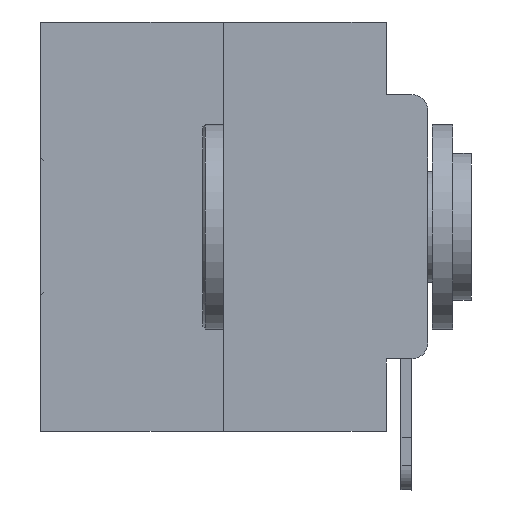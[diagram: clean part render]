
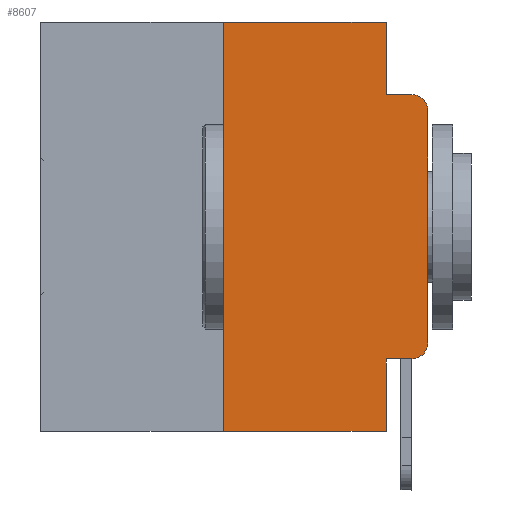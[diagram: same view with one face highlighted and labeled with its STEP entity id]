
A CAD part, left-side view. The second image highlights one B-rep face of the part: STEP entity #8607.
In plain terms, the highlighted planar face has unit normal (-1, 0, 0).
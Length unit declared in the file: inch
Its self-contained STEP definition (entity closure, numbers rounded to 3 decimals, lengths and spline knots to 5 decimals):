
#262 = DIRECTION ( 'NONE',  ( 0., 0., -1. ) ) ;
#319 = CARTESIAN_POINT ( 'NONE',  ( 0., 0.051, -0.4115 ) ) ;
#402 = FACE_OUTER_BOUND ( 'NONE', #17905, .T. ) ;
#576 = LINE ( 'NONE', #646, #9489 ) ;
#646 = CARTESIAN_POINT ( 'NONE',  ( 0., 0.051, -0.0885 ) ) ;
#728 = DIRECTION ( 'NONE',  ( 0., 0., -1. ) ) ;
#1048 = ORIENTED_EDGE ( 'NONE', *, *, #15863, .F. ) ;
#1178 = EDGE_CURVE ( 'NONE', #18117, #3044, #16534, .T. ) ;
#1438 = CARTESIAN_POINT ( 'NONE',  ( 0., 0.25, 0. ) ) ;
#1987 = CARTESIAN_POINT ( 'NONE',  ( 0., 0., -0.1085 ) ) ;
#3044 = VERTEX_POINT ( 'NONE', #31222 ) ;
#3972 = DIRECTION ( 'NONE',  ( 0., -1., 0. ) ) ;
#4255 = EDGE_CURVE ( 'NONE', #9255, #8906, #14794, .T. ) ;
#4724 = CARTESIAN_POINT ( 'NONE',  ( 0., 0.25, -0.5 ) ) ;
#5459 = ORIENTED_EDGE ( 'NONE', *, *, #26812, .T. ) ;
#5686 = DIRECTION ( 'NONE',  ( -1., 0., 0. ) ) ;
#6007 = CARTESIAN_POINT ( 'NONE',  ( 0., 0.02, -0.1085 ) ) ;
#6396 = DIRECTION ( 'NONE',  ( 0., -1., 0. ) ) ;
#6477 = CARTESIAN_POINT ( 'NONE',  ( 0., 0., -0.3915 ) ) ;
#6578 = VECTOR ( 'NONE', #6396, 39.37008 ) ;
#6749 = LINE ( 'NONE', #26304, #31237 ) ;
#7084 = DIRECTION ( 'NONE',  ( 0., 0., -1. ) ) ;
#7358 = AXIS2_PLACEMENT_3D ( 'NONE', #6007, #5686, #728 ) ;
#7733 = ORIENTED_EDGE ( 'NONE', *, *, #22072, .F. ) ;
#7742 = VECTOR ( 'NONE', #15112, 39.37008 ) ;
#8607 = ADVANCED_FACE ( 'NONE', ( #402 ), #12983, .F. ) ;
#8906 = VERTEX_POINT ( 'NONE', #23309 ) ;
#9255 = VERTEX_POINT ( 'NONE', #29209 ) ;
#9489 = VECTOR ( 'NONE', #23239, 39.37008 ) ;
#9783 = VERTEX_POINT ( 'NONE', #6477 ) ;
#9845 = CARTESIAN_POINT ( 'NONE',  ( 0., 0.02, -0.0885 ) ) ;
#10100 = VERTEX_POINT ( 'NONE', #9845 ) ;
#10131 = CARTESIAN_POINT ( 'NONE',  ( 0., 0.473, 0. ) ) ;
#10778 = ORIENTED_EDGE ( 'NONE', *, *, #4255, .F. ) ;
#11889 = AXIS2_PLACEMENT_3D ( 'NONE', #16993, #19528, #7084 ) ;
#12983 = PLANE ( 'NONE',  #27337 ) ;
#13400 = CARTESIAN_POINT ( 'NONE',  ( 0., 0.473, 0. ) ) ;
#13422 = VERTEX_POINT ( 'NONE', #15298 ) ;
#13876 = LINE ( 'NONE', #30488, #19703 ) ;
#14374 = LINE ( 'NONE', #20135, #7742 ) ;
#14794 = LINE ( 'NONE', #17835, #16333 ) ;
#15103 = ORIENTED_EDGE ( 'NONE', *, *, #26096, .T. ) ;
#15112 = DIRECTION ( 'NONE',  ( 0., 0., -1. ) ) ;
#15298 = CARTESIAN_POINT ( 'NONE',  ( 0., 0.051, 0. ) ) ;
#15502 = DIRECTION ( 'NONE',  ( 0., -1., 0. ) ) ;
#15570 = LINE ( 'NONE', #13400, #6578 ) ;
#15663 = DIRECTION ( 'NONE',  ( 0., 0., 1. ) ) ;
#15863 = EDGE_CURVE ( 'NONE', #27999, #10100, #576, .T. ) ;
#16333 = VECTOR ( 'NONE', #262, 39.37008 ) ;
#16534 = LINE ( 'NONE', #1438, #26199 ) ;
#16773 = EDGE_CURVE ( 'NONE', #9783, #29771, #13876, .T. ) ;
#16993 = CARTESIAN_POINT ( 'NONE',  ( 0., 0.02, -0.3915 ) ) ;
#17084 = EDGE_CURVE ( 'NONE', #13422, #27999, #14374, .T. ) ;
#17223 = ORIENTED_EDGE ( 'NONE', *, *, #1178, .F. ) ;
#17383 = LINE ( 'NONE', #319, #27822 ) ;
#17763 = CIRCLE ( 'NONE', #11889, 0.02 ) ;
#17835 = CARTESIAN_POINT ( 'NONE',  ( 0., 0.051, 0. ) ) ;
#17905 = EDGE_LOOP ( 'NONE', ( #20429, #27371, #1048, #22191, #7733, #17223, #5459, #10778, #30061, #15103 ) ) ;
#18117 = VERTEX_POINT ( 'NONE', #4724 ) ;
#19135 = EDGE_CURVE ( 'NONE', #29771, #10100, #30495, .T. ) ;
#19528 = DIRECTION ( 'NONE',  ( -1., 0., 0. ) ) ;
#19703 = VECTOR ( 'NONE', #15663, 39.37008 ) ;
#20135 = CARTESIAN_POINT ( 'NONE',  ( 0., 0.051, 0. ) ) ;
#20429 = ORIENTED_EDGE ( 'NONE', *, *, #16773, .T. ) ;
#22072 = EDGE_CURVE ( 'NONE', #3044, #13422, #15570, .T. ) ;
#22191 = ORIENTED_EDGE ( 'NONE', *, *, #17084, .F. ) ;
#23239 = DIRECTION ( 'NONE',  ( 0., -1., 0. ) ) ;
#23309 = CARTESIAN_POINT ( 'NONE',  ( 0., 0.051, -0.5 ) ) ;
#23918 = CARTESIAN_POINT ( 'NONE',  ( 0., 0.051, -0.0885 ) ) ;
#25320 = DIRECTION ( 'NONE',  ( 0., 0., -1. ) ) ;
#25751 = EDGE_CURVE ( 'NONE', #9255, #31777, #17383, .T. ) ;
#26096 = EDGE_CURVE ( 'NONE', #31777, #9783, #17763, .T. ) ;
#26199 = VECTOR ( 'NONE', #31258, 39.37008 ) ;
#26304 = CARTESIAN_POINT ( 'NONE',  ( 0., 0.473, -0.5 ) ) ;
#26812 = EDGE_CURVE ( 'NONE', #18117, #8906, #6749, .T. ) ;
#27337 = AXIS2_PLACEMENT_3D ( 'NONE', #10131, #29887, #25320 ) ;
#27371 = ORIENTED_EDGE ( 'NONE', *, *, #19135, .T. ) ;
#27664 = CARTESIAN_POINT ( 'NONE',  ( 0., 0.02, -0.4115 ) ) ;
#27822 = VECTOR ( 'NONE', #15502, 39.37008 ) ;
#27999 = VERTEX_POINT ( 'NONE', #23918 ) ;
#29209 = CARTESIAN_POINT ( 'NONE',  ( 0., 0.051, -0.4115 ) ) ;
#29771 = VERTEX_POINT ( 'NONE', #1987 ) ;
#29887 = DIRECTION ( 'NONE',  ( 1., 0., 0. ) ) ;
#30061 = ORIENTED_EDGE ( 'NONE', *, *, #25751, .T. ) ;
#30488 = CARTESIAN_POINT ( 'NONE',  ( 0., 0., 0. ) ) ;
#30495 = CIRCLE ( 'NONE', #7358, 0.02 ) ;
#31222 = CARTESIAN_POINT ( 'NONE',  ( 0., 0.25, 0. ) ) ;
#31237 = VECTOR ( 'NONE', #3972, 39.37008 ) ;
#31258 = DIRECTION ( 'NONE',  ( 0., 0., 1. ) ) ;
#31777 = VERTEX_POINT ( 'NONE', #27664 ) ;
